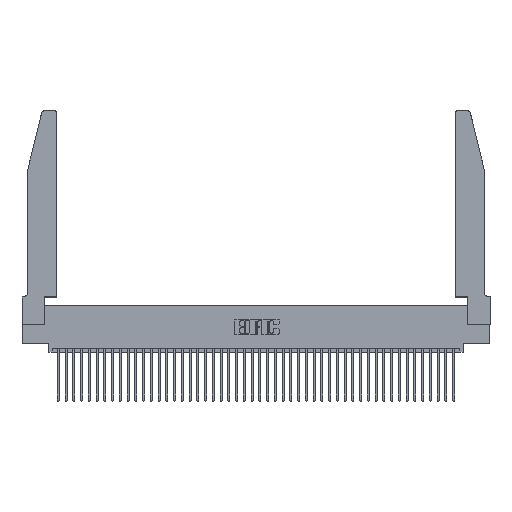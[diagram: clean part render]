
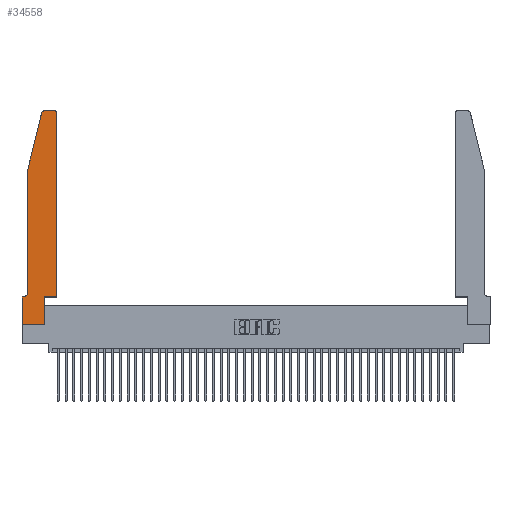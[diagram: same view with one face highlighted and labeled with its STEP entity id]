
A CAD part, top view. The second image highlights one B-rep face of the part: STEP entity #34558.
In plain terms, the highlighted planar face has unit normal (0, 0, 1).
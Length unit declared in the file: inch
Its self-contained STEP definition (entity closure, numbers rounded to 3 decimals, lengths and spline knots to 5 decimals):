
#27 = VERTEX_POINT ( 'NONE', #5205 ) ;
#276 = VERTEX_POINT ( 'NONE', #11237 ) ;
#390 = ORIENTED_EDGE ( 'NONE', *, *, #19505, .T. ) ;
#1003 = LINE ( 'NONE', #15913, #31135 ) ;
#1181 = VERTEX_POINT ( 'NONE', #14981 ) ;
#1429 = DIRECTION ( 'NONE',  ( 0., 1., 0. ) ) ;
#1854 = LINE ( 'NONE', #16359, #11549 ) ;
#2233 = CARTESIAN_POINT ( 'NONE',  ( 0.0755, 2., 0.37 ) ) ;
#2379 = CARTESIAN_POINT ( 'NONE',  ( 0.0055, 0.35, 0.37 ) ) ;
#2463 = ORIENTED_EDGE ( 'NONE', *, *, #29017, .T. ) ;
#3958 = VERTEX_POINT ( 'NONE', #10244 ) ;
#4793 = LINE ( 'NONE', #29080, #31656 ) ;
#5205 = CARTESIAN_POINT ( 'NONE',  ( 0., 0.35, 0.37 ) ) ;
#5849 = DIRECTION ( 'NONE',  ( -1., 0., 0. ) ) ;
#6182 = LINE ( 'NONE', #32740, #7229 ) ;
#6276 = CARTESIAN_POINT ( 'NONE',  ( 0.0055, 0.42, 0.37 ) ) ;
#6437 = EDGE_CURVE ( 'NONE', #27275, #40441, #11055, .T. ) ;
#7229 = VECTOR ( 'NONE', #32888, 39.37008 ) ;
#8096 = ORIENTED_EDGE ( 'NONE', *, *, #12906, .T. ) ;
#8155 = DIRECTION ( 'NONE',  ( 0., 0., 1. ) ) ;
#8514 = ORIENTED_EDGE ( 'NONE', *, *, #13282, .T. ) ;
#9148 = CIRCLE ( 'NONE', #15169, 0.03 ) ;
#10081 = VERTEX_POINT ( 'NONE', #31389 ) ;
#10244 = CARTESIAN_POINT ( 'NONE',  ( 0.4505, 2.72, 0.37 ) ) ;
#11055 = CIRCLE ( 'NONE', #33871, 0.07 ) ;
#11063 = ORIENTED_EDGE ( 'NONE', *, *, #17620, .T. ) ;
#11237 = CARTESIAN_POINT ( 'NONE',  ( 0.2865, 0.35, 0.37 ) ) ;
#11285 = CARTESIAN_POINT ( 'NONE',  ( 0.0755, 0.42, 0.37 ) ) ;
#11443 = EDGE_LOOP ( 'NONE', ( #37519, #26876, #11063, #390, #41015, #8514, #39088, #16190, #38739, #2463, #25532, #8096 ) ) ;
#11549 = VECTOR ( 'NONE', #15921, 39.37008 ) ;
#12802 = CARTESIAN_POINT ( 'NONE',  ( 0.0755, 2., 0.37 ) ) ;
#12906 = EDGE_CURVE ( 'NONE', #3958, #29859, #15362, .T. ) ;
#13002 = VECTOR ( 'NONE', #39128, 39.37008 ) ;
#13075 = VERTEX_POINT ( 'NONE', #21905 ) ;
#13282 = EDGE_CURVE ( 'NONE', #40441, #27, #1854, .T. ) ;
#14341 = LINE ( 'NONE', #25132, #23557 ) ;
#14759 = DIRECTION ( 'NONE',  ( 0., 0., 1. ) ) ;
#14981 = CARTESIAN_POINT ( 'NONE',  ( 0.284, 2.75, 0.37 ) ) ;
#15169 = AXIS2_PLACEMENT_3D ( 'NONE', #24992, #14759, #21071 ) ;
#15362 = CIRCLE ( 'NONE', #21316, 0.03 ) ;
#15913 = CARTESIAN_POINT ( 'NONE',  ( 0., 0., 0.37 ) ) ;
#15921 = DIRECTION ( 'NONE',  ( -1., 0., 0. ) ) ;
#16190 = ORIENTED_EDGE ( 'NONE', *, *, #31983, .T. ) ;
#16359 = CARTESIAN_POINT ( 'NONE',  ( 0.0755, 0.35, 0.37 ) ) ;
#17449 = FACE_OUTER_BOUND ( 'NONE', #11443, .T. ) ;
#17620 = EDGE_CURVE ( 'NONE', #41849, #10081, #22160, .T. ) ;
#17844 = VECTOR ( 'NONE', #27831, 39.37008 ) ;
#18539 = DIRECTION ( 'NONE',  ( 1., 0., 0. ) ) ;
#18878 = DIRECTION ( 'NONE',  ( 1., 0., 0. ) ) ;
#19505 = EDGE_CURVE ( 'NONE', #10081, #27275, #39678, .T. ) ;
#20175 = AXIS2_PLACEMENT_3D ( 'NONE', #38979, #22046, #18878 ) ;
#20332 = EDGE_CURVE ( 'NONE', #29859, #1181, #14341, .T. ) ;
#20997 = VERTEX_POINT ( 'NONE', #26335 ) ;
#21071 = DIRECTION ( 'NONE',  ( 1., 0., 0. ) ) ;
#21316 = AXIS2_PLACEMENT_3D ( 'NONE', #21685, #8155, #18539 ) ;
#21685 = CARTESIAN_POINT ( 'NONE',  ( 0.4205, 2.72, 0.37 ) ) ;
#21905 = CARTESIAN_POINT ( 'NONE',  ( 0.2865, 0., 0.37 ) ) ;
#22046 = DIRECTION ( 'NONE',  ( 0., 0., 1. ) ) ;
#22160 = LINE ( 'NONE', #2233, #13002 ) ;
#23508 = DIRECTION ( 'NONE',  ( 1., 0., 0. ) ) ;
#23557 = VECTOR ( 'NONE', #28567, 39.37008 ) ;
#24992 = CARTESIAN_POINT ( 'NONE',  ( 0.284, 2.72, 0.37 ) ) ;
#25132 = CARTESIAN_POINT ( 'NONE',  ( 0.2605, 2.75, 0.37 ) ) ;
#25532 = ORIENTED_EDGE ( 'NONE', *, *, #26540, .T. ) ;
#26335 = CARTESIAN_POINT ( 'NONE',  ( 0.4505, 0.35, 0.37 ) ) ;
#26518 = CARTESIAN_POINT ( 'NONE',  ( 0.4505, 0.35, 0.37 ) ) ;
#26540 = EDGE_CURVE ( 'NONE', #20997, #3958, #4793, .T. ) ;
#26579 = DIRECTION ( 'NONE',  ( 1., 0., 0. ) ) ;
#26876 = ORIENTED_EDGE ( 'NONE', *, *, #39398, .T. ) ;
#26923 = DIRECTION ( 'NONE',  ( 0., -1., 0. ) ) ;
#27275 = VERTEX_POINT ( 'NONE', #11285 ) ;
#27831 = DIRECTION ( 'NONE',  ( 0., 1., 0. ) ) ;
#28567 = DIRECTION ( 'NONE',  ( -1., 0., 0. ) ) ;
#29017 = EDGE_CURVE ( 'NONE', #276, #20997, #30359, .T. ) ;
#29080 = CARTESIAN_POINT ( 'NONE',  ( 0.4505, 0.35, 0.37 ) ) ;
#29859 = VERTEX_POINT ( 'NONE', #38719 ) ;
#30359 = LINE ( 'NONE', #26518, #33053 ) ;
#31135 = VECTOR ( 'NONE', #26579, 39.37008 ) ;
#31389 = CARTESIAN_POINT ( 'NONE',  ( 0.0755, 2., 0.37 ) ) ;
#31447 = CARTESIAN_POINT ( 'NONE',  ( 0.2865, 0.35, 0.37 ) ) ;
#31656 = VECTOR ( 'NONE', #1429, 39.37008 ) ;
#31983 = EDGE_CURVE ( 'NONE', #38281, #13075, #1003, .T. ) ;
#32740 = CARTESIAN_POINT ( 'NONE',  ( 0., 0., 0.37 ) ) ;
#32888 = DIRECTION ( 'NONE',  ( 0., -1., 0. ) ) ;
#33053 = VECTOR ( 'NONE', #23508, 39.37008 ) ;
#33871 = AXIS2_PLACEMENT_3D ( 'NONE', #6276, #43925, #5849 ) ;
#34017 = CARTESIAN_POINT ( 'NONE',  ( 0., 0., 0.37 ) ) ;
#34558 = ADVANCED_FACE ( 'NONE', ( #17449 ), #39284, .T. ) ;
#35596 = EDGE_CURVE ( 'NONE', #13075, #276, #38284, .T. ) ;
#37519 = ORIENTED_EDGE ( 'NONE', *, *, #20332, .T. ) ;
#38281 = VERTEX_POINT ( 'NONE', #34017 ) ;
#38284 = LINE ( 'NONE', #31447, #17844 ) ;
#38719 = CARTESIAN_POINT ( 'NONE',  ( 0.4205, 2.75, 0.37 ) ) ;
#38739 = ORIENTED_EDGE ( 'NONE', *, *, #35596, .T. ) ;
#38979 = CARTESIAN_POINT ( 'NONE',  ( 0., 0.35, 0.37 ) ) ;
#39088 = ORIENTED_EDGE ( 'NONE', *, *, #42513, .T. ) ;
#39128 = DIRECTION ( 'NONE',  ( -0.239, -0.971, 0. ) ) ;
#39284 = PLANE ( 'NONE',  #20175 ) ;
#39398 = EDGE_CURVE ( 'NONE', #1181, #41849, #9148, .T. ) ;
#39678 = LINE ( 'NONE', #12802, #43929 ) ;
#40441 = VERTEX_POINT ( 'NONE', #2379 ) ;
#41015 = ORIENTED_EDGE ( 'NONE', *, *, #6437, .T. ) ;
#41849 = VERTEX_POINT ( 'NONE', #42324 ) ;
#42324 = CARTESIAN_POINT ( 'NONE',  ( 0.25487, 2.72718, 0.37 ) ) ;
#42513 = EDGE_CURVE ( 'NONE', #27, #38281, #6182, .T. ) ;
#43925 = DIRECTION ( 'NONE',  ( 0., 0., -1. ) ) ;
#43929 = VECTOR ( 'NONE', #26923, 39.37008 ) ;
